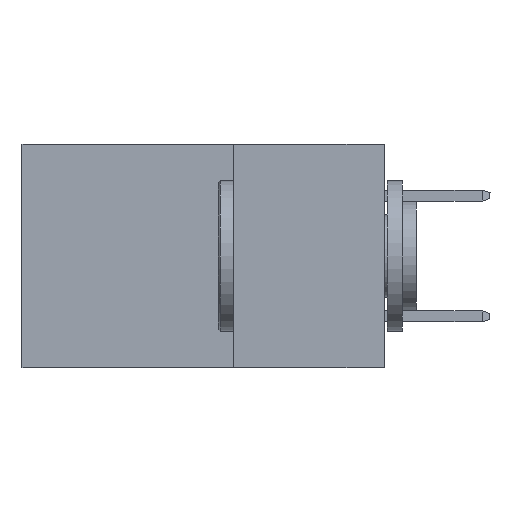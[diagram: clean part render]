
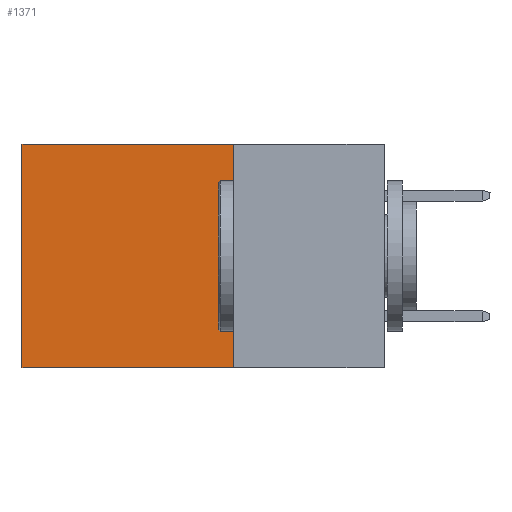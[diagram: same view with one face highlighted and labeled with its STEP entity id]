
A CAD part, left-side view. The second image highlights one B-rep face of the part: STEP entity #1371.
In plain terms, the highlighted planar face has unit normal (-1, 0, 0).
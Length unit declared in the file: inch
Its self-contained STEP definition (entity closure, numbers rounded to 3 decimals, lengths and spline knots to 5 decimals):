
#12 = CARTESIAN_POINT ( 'NONE',  ( 0.2615, 0.25, 0. ) ) ;
#1111 = DIRECTION ( 'NONE',  ( 0., 1., 0. ) ) ;
#1121 = LINE ( 'NONE', #22585, #5156 ) ;
#1371 = ADVANCED_FACE ( 'NONE', ( #14909 ), #16391, .F. ) ;
#2192 = EDGE_CURVE ( 'NONE', #3426, #8426, #1121, .T. ) ;
#2256 = VECTOR ( 'NONE', #1111, 39.37008 ) ;
#3426 = VERTEX_POINT ( 'NONE', #10908 ) ;
#4817 = LINE ( 'NONE', #19248, #22606 ) ;
#5156 = VECTOR ( 'NONE', #22485, 39.37008 ) ;
#5747 = ORIENTED_EDGE ( 'NONE', *, *, #14364, .F. ) ;
#6487 = VERTEX_POINT ( 'NONE', #12 ) ;
#6898 = ORIENTED_EDGE ( 'NONE', *, *, #2192, .T. ) ;
#8426 = VERTEX_POINT ( 'NONE', #10574 ) ;
#9044 = DIRECTION ( 'NONE',  ( 0., 0., -1. ) ) ;
#9553 = ORIENTED_EDGE ( 'NONE', *, *, #14256, .T. ) ;
#10466 = DIRECTION ( 'NONE',  ( 0., 1., 0. ) ) ;
#10574 = CARTESIAN_POINT ( 'NONE',  ( 0.2615, 0.6, -0.37 ) ) ;
#10634 = EDGE_LOOP ( 'NONE', ( #6898, #5747, #17170, #9553 ) ) ;
#10908 = CARTESIAN_POINT ( 'NONE',  ( 0.2615, 0.6, 0. ) ) ;
#11281 = LINE ( 'NONE', #22503, #2256 ) ;
#13376 = VERTEX_POINT ( 'NONE', #21993 ) ;
#13978 = VECTOR ( 'NONE', #9044, 39.37008 ) ;
#14256 = EDGE_CURVE ( 'NONE', #6487, #3426, #11281, .T. ) ;
#14364 = EDGE_CURVE ( 'NONE', #13376, #8426, #4817, .T. ) ;
#14909 = FACE_OUTER_BOUND ( 'NONE', #10634, .T. ) ;
#15751 = EDGE_CURVE ( 'NONE', #6487, #13376, #22864, .T. ) ;
#16248 = CARTESIAN_POINT ( 'NONE',  ( 0.2615, 0.25, -0.37 ) ) ;
#16391 = PLANE ( 'NONE',  #21567 ) ;
#17170 = ORIENTED_EDGE ( 'NONE', *, *, #15751, .F. ) ;
#17877 = DIRECTION ( 'NONE',  ( 0., 0., -1. ) ) ;
#17933 = DIRECTION ( 'NONE',  ( 1., 0., 0. ) ) ;
#19248 = CARTESIAN_POINT ( 'NONE',  ( 0.2615, 0.25, -0.37 ) ) ;
#21365 = CARTESIAN_POINT ( 'NONE',  ( 0.2615, 0.25, -0.37 ) ) ;
#21567 = AXIS2_PLACEMENT_3D ( 'NONE', #16248, #17933, #17877 ) ;
#21993 = CARTESIAN_POINT ( 'NONE',  ( 0.2615, 0.25, -0.37 ) ) ;
#22485 = DIRECTION ( 'NONE',  ( 0., 0., -1. ) ) ;
#22503 = CARTESIAN_POINT ( 'NONE',  ( 0.2615, 0.25, 0. ) ) ;
#22585 = CARTESIAN_POINT ( 'NONE',  ( 0.2615, 0.6, -0.37 ) ) ;
#22606 = VECTOR ( 'NONE', #10466, 39.37008 ) ;
#22864 = LINE ( 'NONE', #21365, #13978 ) ;
